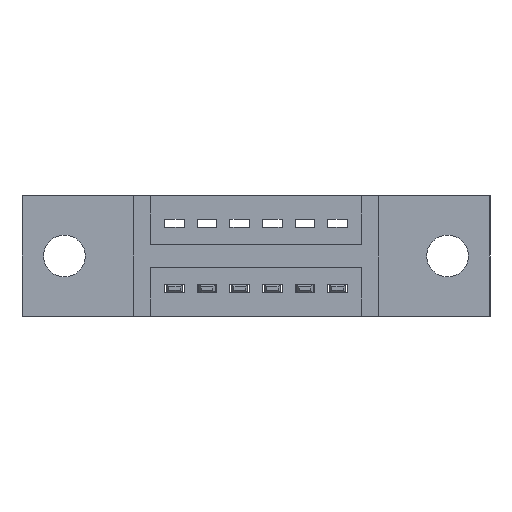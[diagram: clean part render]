
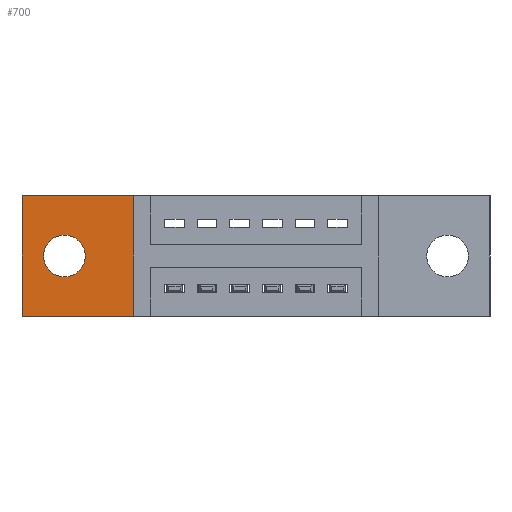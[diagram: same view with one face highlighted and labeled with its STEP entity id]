
A CAD part, front view. The second image highlights one B-rep face of the part: STEP entity #700.
In plain terms, the highlighted planar face has unit normal (0, -1, 0).
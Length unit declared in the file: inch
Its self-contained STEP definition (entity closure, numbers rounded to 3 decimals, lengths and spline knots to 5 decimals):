
#507 = VERTEX_POINT ( 'NONE', #3797 ) ;
#568 = DIRECTION ( 'NONE',  ( -1., 0., 0. ) ) ;
#580 = DIRECTION ( 'NONE',  ( 0., -1., 0. ) ) ;
#700 = ADVANCED_FACE ( 'NONE', ( #6209, #5216 ), #8389, .T. ) ;
#1276 = CARTESIAN_POINT ( 'NONE',  ( 0.13, 0.17, -0.185 ) ) ;
#1303 = DIRECTION ( 'NONE',  ( 0., -1., 0. ) ) ;
#1538 = VERTEX_POINT ( 'NONE', #2010 ) ;
#2010 = CARTESIAN_POINT ( 'NONE',  ( 0.3425, 0.17, 0. ) ) ;
#2218 = LINE ( 'NONE', #7206, #5267 ) ;
#2287 = CARTESIAN_POINT ( 'NONE',  ( 0., 0.17, -0.37 ) ) ;
#2733 = DIRECTION ( 'NONE',  ( 0., 0., -1. ) ) ;
#3403 = DIRECTION ( 'NONE',  ( 0., 0., -1. ) ) ;
#3563 = EDGE_CURVE ( 'NONE', #1538, #6798, #7193, .T. ) ;
#3634 = CARTESIAN_POINT ( 'NONE',  ( 0., 0.17, 0. ) ) ;
#3640 = CARTESIAN_POINT ( 'NONE',  ( 0., 0.17, 0. ) ) ;
#3797 = CARTESIAN_POINT ( 'NONE',  ( 0.13, 0.17, -0.121 ) ) ;
#4047 = DIRECTION ( 'NONE',  ( 0., -1., 0. ) ) ;
#4254 = ORIENTED_EDGE ( 'NONE', *, *, #3563, .T. ) ;
#4350 = CARTESIAN_POINT ( 'NONE',  ( 0.3425, 0.17, -0.37 ) ) ;
#4628 = DIRECTION ( 'NONE',  ( 0., 0., 1. ) ) ;
#4645 = EDGE_LOOP ( 'NONE', ( #7446, #5343 ) ) ;
#4717 = CARTESIAN_POINT ( 'NONE',  ( 0.3425, 0.17, 0. ) ) ;
#4747 = CARTESIAN_POINT ( 'NONE',  ( 0.13, 0.17, -0.185 ) ) ;
#4788 = VECTOR ( 'NONE', #4628, 39.37008 ) ;
#4887 = CARTESIAN_POINT ( 'NONE',  ( 0., 0.17, 0. ) ) ;
#5216 = FACE_OUTER_BOUND ( 'NONE', #6937, .T. ) ;
#5267 = VECTOR ( 'NONE', #9207, 39.37008 ) ;
#5297 = AXIS2_PLACEMENT_3D ( 'NONE', #1276, #580, #3403 ) ;
#5325 = ORIENTED_EDGE ( 'NONE', *, *, #7356, .T. ) ;
#5343 = ORIENTED_EDGE ( 'NONE', *, *, #5971, .F. ) ;
#5617 = LINE ( 'NONE', #3634, #5952 ) ;
#5952 = VECTOR ( 'NONE', #7969, 39.37008 ) ;
#5971 = EDGE_CURVE ( 'NONE', #5992, #507, #6183, .T. ) ;
#5992 = VERTEX_POINT ( 'NONE', #7006 ) ;
#6183 = CIRCLE ( 'NONE', #5297, 0.064 ) ;
#6203 = DIRECTION ( 'NONE',  ( 0., 0., -1. ) ) ;
#6209 = FACE_BOUND ( 'NONE', #4645, .T. ) ;
#6798 = VERTEX_POINT ( 'NONE', #3640 ) ;
#6830 = ORIENTED_EDGE ( 'NONE', *, *, #8165, .T. ) ;
#6884 = VERTEX_POINT ( 'NONE', #2287 ) ;
#6937 = EDGE_LOOP ( 'NONE', ( #5325, #7911, #6830, #4254 ) ) ;
#7006 = CARTESIAN_POINT ( 'NONE',  ( 0.13, 0.17, -0.249 ) ) ;
#7193 = LINE ( 'NONE', #4887, #7731 ) ;
#7206 = CARTESIAN_POINT ( 'NONE',  ( 0., 0.17, -0.37 ) ) ;
#7356 = EDGE_CURVE ( 'NONE', #6798, #6884, #5617, .T. ) ;
#7364 = VERTEX_POINT ( 'NONE', #4350 ) ;
#7392 = LINE ( 'NONE', #4717, #4788 ) ;
#7446 = ORIENTED_EDGE ( 'NONE', *, *, #8649, .F. ) ;
#7499 = CIRCLE ( 'NONE', #9026, 0.064 ) ;
#7731 = VECTOR ( 'NONE', #568, 39.37008 ) ;
#7747 = CARTESIAN_POINT ( 'NONE',  ( 0., 0.17, -0.37 ) ) ;
#7821 = EDGE_CURVE ( 'NONE', #6884, #7364, #2218, .T. ) ;
#7911 = ORIENTED_EDGE ( 'NONE', *, *, #7821, .T. ) ;
#7969 = DIRECTION ( 'NONE',  ( 0., 0., -1. ) ) ;
#8165 = EDGE_CURVE ( 'NONE', #7364, #1538, #7392, .T. ) ;
#8389 = PLANE ( 'NONE',  #8686 ) ;
#8649 = EDGE_CURVE ( 'NONE', #507, #5992, #7499, .T. ) ;
#8686 = AXIS2_PLACEMENT_3D ( 'NONE', #7747, #1303, #2733 ) ;
#9026 = AXIS2_PLACEMENT_3D ( 'NONE', #4747, #4047, #6203 ) ;
#9207 = DIRECTION ( 'NONE',  ( 1., 0., 0. ) ) ;
